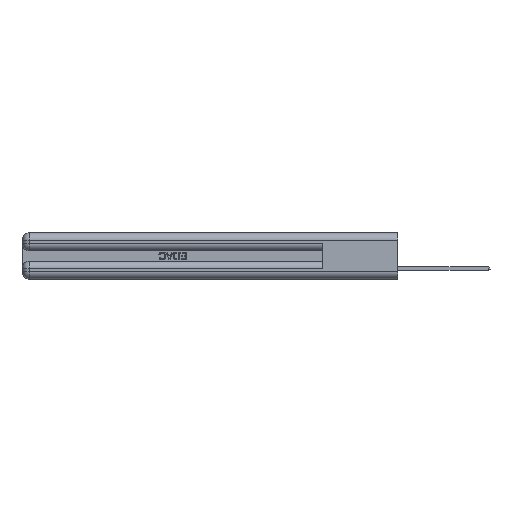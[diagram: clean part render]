
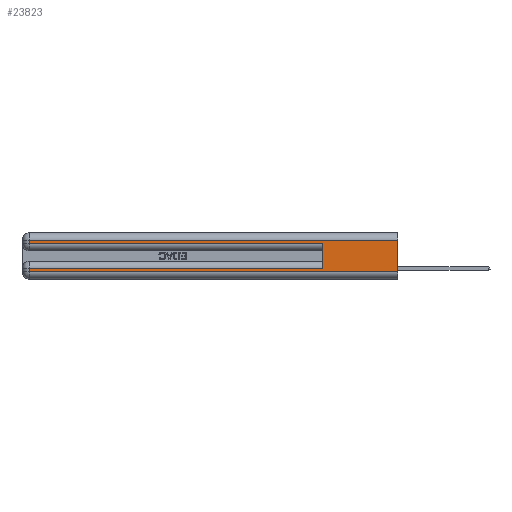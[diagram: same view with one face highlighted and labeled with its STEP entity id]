
A CAD part, left-side view. The second image highlights one B-rep face of the part: STEP entity #23823.
In plain terms, the highlighted planar face has unit normal (-1, 0, 0).
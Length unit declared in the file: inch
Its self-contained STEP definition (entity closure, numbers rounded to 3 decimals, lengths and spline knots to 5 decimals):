
#386 = CARTESIAN_POINT ( 'NONE',  ( 0., 0.6, 0.145 ) ) ;
#943 = FACE_OUTER_BOUND ( 'NONE', #40442, .T. ) ;
#1580 = LINE ( 'NONE', #19849, #26177 ) ;
#2326 = VERTEX_POINT ( 'NONE', #29882 ) ;
#2625 = CARTESIAN_POINT ( 'NONE',  ( 0., 2.94, 0.37 ) ) ;
#3645 = EDGE_CURVE ( 'NONE', #13662, #13085, #42982, .T. ) ;
#3806 = ORIENTED_EDGE ( 'NONE', *, *, #26013, .T. ) ;
#4082 = ORIENTED_EDGE ( 'NONE', *, *, #20123, .T. ) ;
#4904 = LINE ( 'NONE', #8585, #21393 ) ;
#5064 = AXIS2_PLACEMENT_3D ( 'NONE', #9289, #13395, #46056 ) ;
#8163 = LINE ( 'NONE', #15011, #51836 ) ;
#8585 = CARTESIAN_POINT ( 'NONE',  ( 0., 0., 0.06 ) ) ;
#9289 = CARTESIAN_POINT ( 'NONE',  ( 0., 0., 0.37 ) ) ;
#10546 = CARTESIAN_POINT ( 'NONE',  ( 0., 2.94, 0.085 ) ) ;
#12751 = DIRECTION ( 'NONE',  ( 0., 0., 1. ) ) ;
#13085 = VERTEX_POINT ( 'NONE', #37156 ) ;
#13335 = LINE ( 'NONE', #26570, #26622 ) ;
#13395 = DIRECTION ( 'NONE',  ( 1., 0., 0. ) ) ;
#13662 = VERTEX_POINT ( 'NONE', #37322 ) ;
#15011 = CARTESIAN_POINT ( 'NONE',  ( 0., 2.94, 0.37 ) ) ;
#15763 = DIRECTION ( 'NONE',  ( 0., -1., 0. ) ) ;
#16613 = CARTESIAN_POINT ( 'NONE',  ( 0., 2.94, 0.06 ) ) ;
#16938 = DIRECTION ( 'NONE',  ( 0., -1., 0. ) ) ;
#16974 = VECTOR ( 'NONE', #12751, 39.37008 ) ;
#19849 = CARTESIAN_POINT ( 'NONE',  ( 0., 0., 0.285 ) ) ;
#20123 = EDGE_CURVE ( 'NONE', #13662, #40702, #38016, .T. ) ;
#20308 = VECTOR ( 'NONE', #39086, 39.37008 ) ;
#21393 = VECTOR ( 'NONE', #16938, 39.37008 ) ;
#21472 = CARTESIAN_POINT ( 'NONE',  ( 0., 2.94, 0.31 ) ) ;
#22650 = CARTESIAN_POINT ( 'NONE',  ( 0., 0., 0.37 ) ) ;
#23823 = ADVANCED_FACE ( 'NONE', ( #943 ), #41521, .F. ) ;
#26013 = EDGE_CURVE ( 'NONE', #2326, #47634, #13335, .T. ) ;
#26177 = VECTOR ( 'NONE', #15763, 39.37008 ) ;
#26450 = CARTESIAN_POINT ( 'NONE',  ( 0., 0., 0.085 ) ) ;
#26570 = CARTESIAN_POINT ( 'NONE',  ( 0., 0., 0.31 ) ) ;
#26622 = VECTOR ( 'NONE', #39193, 39.37008 ) ;
#26697 = ORIENTED_EDGE ( 'NONE', *, *, #48282, .T. ) ;
#27623 = ORIENTED_EDGE ( 'NONE', *, *, #50032, .T. ) ;
#27637 = ORIENTED_EDGE ( 'NONE', *, *, #3645, .F. ) ;
#27793 = CARTESIAN_POINT ( 'NONE',  ( 0., 2.94, 0.285 ) ) ;
#28544 = ORIENTED_EDGE ( 'NONE', *, *, #40302, .T. ) ;
#28617 = EDGE_CURVE ( 'NONE', #2326, #51746, #31029, .T. ) ;
#29882 = CARTESIAN_POINT ( 'NONE',  ( 0., 0., 0.31 ) ) ;
#31029 = LINE ( 'NONE', #22650, #20308 ) ;
#31051 = DIRECTION ( 'NONE',  ( 0., 0., -1. ) ) ;
#31233 = VECTOR ( 'NONE', #31051, 39.37008 ) ;
#32468 = LINE ( 'NONE', #2625, #31233 ) ;
#34780 = DIRECTION ( 'NONE',  ( 0., 0., -1. ) ) ;
#35140 = CARTESIAN_POINT ( 'NONE',  ( 0., 0., 0.06 ) ) ;
#37156 = CARTESIAN_POINT ( 'NONE',  ( 0., 0.6, 0.285 ) ) ;
#37322 = CARTESIAN_POINT ( 'NONE',  ( 0., 0.6, 0.085 ) ) ;
#38005 = DIRECTION ( 'NONE',  ( 0., 1., 0. ) ) ;
#38016 = LINE ( 'NONE', #26450, #40546 ) ;
#39086 = DIRECTION ( 'NONE',  ( 0., 0., -1. ) ) ;
#39193 = DIRECTION ( 'NONE',  ( 0., 1., 0. ) ) ;
#40302 = EDGE_CURVE ( 'NONE', #41510, #13085, #1580, .T. ) ;
#40442 = EDGE_LOOP ( 'NONE', ( #45097, #3806, #26697, #28544, #27637, #4082, #27623, #51557 ) ) ;
#40546 = VECTOR ( 'NONE', #38005, 39.37008 ) ;
#40702 = VERTEX_POINT ( 'NONE', #10546 ) ;
#41510 = VERTEX_POINT ( 'NONE', #27793 ) ;
#41521 = PLANE ( 'NONE',  #5064 ) ;
#42982 = LINE ( 'NONE', #386, #16974 ) ;
#43540 = VERTEX_POINT ( 'NONE', #16613 ) ;
#45097 = ORIENTED_EDGE ( 'NONE', *, *, #28617, .F. ) ;
#46056 = DIRECTION ( 'NONE',  ( 0., 0., -1. ) ) ;
#47634 = VERTEX_POINT ( 'NONE', #21472 ) ;
#48282 = EDGE_CURVE ( 'NONE', #47634, #41510, #32468, .T. ) ;
#50032 = EDGE_CURVE ( 'NONE', #40702, #43540, #8163, .T. ) ;
#51239 = EDGE_CURVE ( 'NONE', #43540, #51746, #4904, .T. ) ;
#51557 = ORIENTED_EDGE ( 'NONE', *, *, #51239, .T. ) ;
#51746 = VERTEX_POINT ( 'NONE', #35140 ) ;
#51836 = VECTOR ( 'NONE', #34780, 39.37008 ) ;
